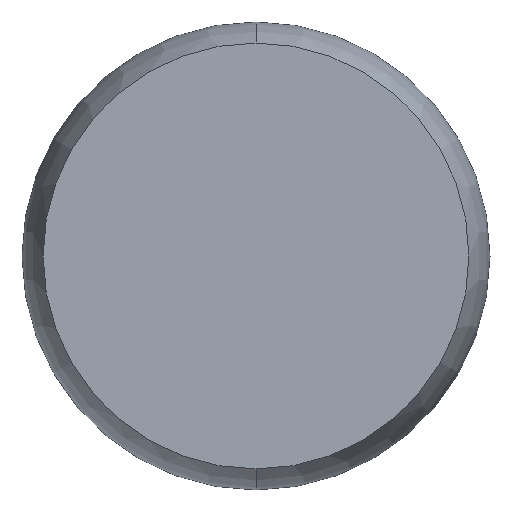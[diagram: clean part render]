
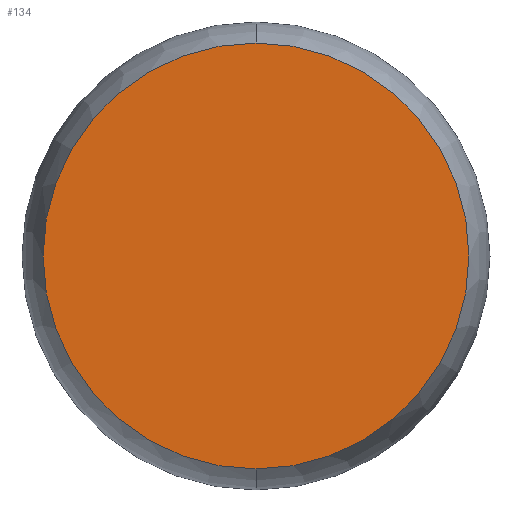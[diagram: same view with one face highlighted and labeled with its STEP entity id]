
A CAD part, front view. The second image highlights one B-rep face of the part: STEP entity #134.
In plain terms, the highlighted planar face has unit normal (0, -1, 0).
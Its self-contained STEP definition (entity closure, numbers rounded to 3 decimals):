
#8 = DIRECTION ( 'NONE',  ( 0., 0., -1. ) ) ;
#10 = DIRECTION ( 'NONE',  ( 0., -1., 0. ) ) ;
#31 = CARTESIAN_POINT ( 'NONE',  ( 0., 0., 0. ) ) ;
#33 = AXIS2_PLACEMENT_3D ( 'NONE', #31, #38, #51 ) ;
#38 = DIRECTION ( 'NONE',  ( 0., -1., 0. ) ) ;
#47 = AXIS2_PLACEMENT_3D ( 'NONE', #151, #10, #8 ) ;
#51 = DIRECTION ( 'NONE',  ( 0., 0., -1. ) ) ;
#52 = AXIS2_PLACEMENT_3D ( 'NONE', #84, #223, #58 ) ;
#58 = DIRECTION ( 'NONE',  ( 0., 0., -1. ) ) ;
#63 = VERTEX_POINT ( 'NONE', #241 ) ;
#75 = EDGE_CURVE ( 'NONE', #63, #111, #88, .T. ) ;
#78 = EDGE_CURVE ( 'NONE', #111, #63, #83, .T. ) ;
#83 = CIRCLE ( 'NONE', #47, 3.797 ) ;
#84 = CARTESIAN_POINT ( 'NONE',  ( 0., 0., 0. ) ) ;
#88 = CIRCLE ( 'NONE', #52, 3.797 ) ;
#111 = VERTEX_POINT ( 'NONE', #173 ) ;
#134 = ADVANCED_FACE ( 'NONE', ( #215 ), #174, .T. ) ;
#149 = EDGE_LOOP ( 'NONE', ( #216, #190 ) ) ;
#151 = CARTESIAN_POINT ( 'NONE',  ( 0., 0., 0. ) ) ;
#173 = CARTESIAN_POINT ( 'NONE',  ( 0., 0., 3.797 ) ) ;
#174 = PLANE ( 'NONE',  #33 ) ;
#190 = ORIENTED_EDGE ( 'NONE', *, *, #78, .T. ) ;
#215 = FACE_OUTER_BOUND ( 'NONE', #149, .T. ) ;
#216 = ORIENTED_EDGE ( 'NONE', *, *, #75, .T. ) ;
#223 = DIRECTION ( 'NONE',  ( 0., -1., 0. ) ) ;
#241 = CARTESIAN_POINT ( 'NONE',  ( 0., 0., -3.797 ) ) ;
